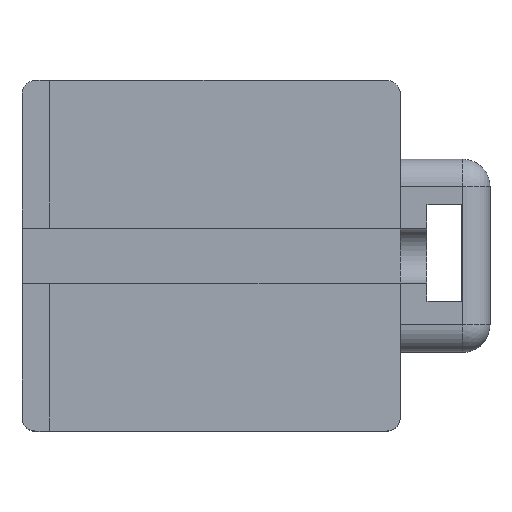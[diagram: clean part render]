
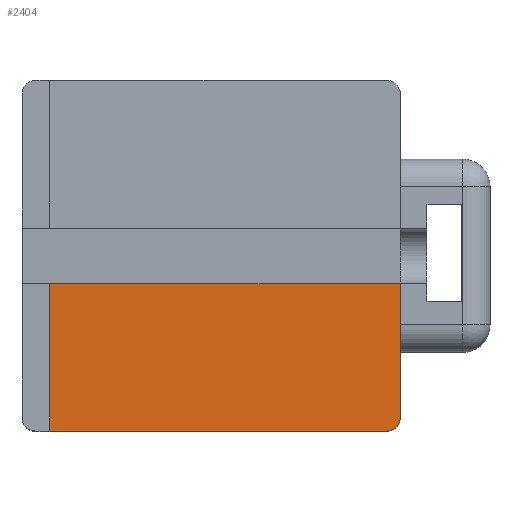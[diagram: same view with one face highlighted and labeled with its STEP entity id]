
A CAD part, top view. The second image highlights one B-rep face of the part: STEP entity #2404.
In plain terms, the highlighted planar face has unit normal (0, 0, 1).
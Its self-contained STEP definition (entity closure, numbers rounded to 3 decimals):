
#599 = PLANE('',#600);
#600 = AXIS2_PLACEMENT_3D('',#601,#602,#603);
#601 = CARTESIAN_POINT('',(4.864,-30.767,17.467));
#602 = DIRECTION('',(1.,0.,0.));
#603 = DIRECTION('',(0.,0.,1.));
#1413 = VERTEX_POINT('',#1414);
#1414 = CARTESIAN_POINT('',(4.864,-14.7,16.036));
#1428 = PLANE('',#1429);
#1429 = AXIS2_PLACEMENT_3D('',#1430,#1431,#1432);
#1430 = CARTESIAN_POINT('',(4.864,-14.7,14.));
#1431 = DIRECTION('',(0.,1.,0.));
#1432 = DIRECTION('',(0.,0.,1.));
#1440 = EDGE_CURVE('',#1441,#1413,#1443,.T.);
#1441 = VERTEX_POINT('',#1442);
#1442 = CARTESIAN_POINT('',(4.864,-24.4,16.036));
#1443 = SURFACE_CURVE('',#1444,(#1448,#1454),.PCURVE_S1.);
#1444 = LINE('',#1445,#1446);
#1445 = CARTESIAN_POINT('',(4.864,-28.084,16.036));
#1446 = VECTOR('',#1447,1.);
#1447 = DIRECTION('',(0.,1.,0.));
#1448 = PCURVE('',#599,#1449);
#1449 = DEFINITIONAL_REPRESENTATION('',(#1450),#1453);
#1450 = B_SPLINE_CURVE_WITH_KNOTS('',1,(#1451,#1452),.UNSPECIFIED.,.F.,
  .F.,(2,2),(0.144,30.624),.PIECEWISE_BEZIER_KNOTS.);
#1451 = CARTESIAN_POINT('',(-1.431,-2.827));
#1452 = CARTESIAN_POINT('',(-1.431,-33.307));
#1453 = ( GEOMETRIC_REPRESENTATION_CONTEXT(2) 
PARAMETRIC_REPRESENTATION_CONTEXT() REPRESENTATION_CONTEXT('2D SPACE',''
  ) );
#1454 = PCURVE('',#1455,#1460);
#1455 = PLANE('',#1456);
#1456 = AXIS2_PLACEMENT_3D('',#1457,#1458,#1459);
#1457 = CARTESIAN_POINT('',(-7.836,-25.4,16.036));
#1458 = DIRECTION('',(0.,0.,1.));
#1459 = DIRECTION('',(0.,-1.,0.));
#1460 = DEFINITIONAL_REPRESENTATION('',(#1461),#1464);
#1461 = B_SPLINE_CURVE_WITH_KNOTS('',1,(#1462,#1463),.UNSPECIFIED.,.F.,
  .F.,(2,2),(0.144,30.624),.PIECEWISE_BEZIER_KNOTS.);
#1462 = CARTESIAN_POINT('',(2.54,12.7));
#1463 = CARTESIAN_POINT('',(-27.94,12.7));
#1464 = ( GEOMETRIC_REPRESENTATION_CONTEXT(2) 
PARAMETRIC_REPRESENTATION_CONTEXT() REPRESENTATION_CONTEXT('2D SPACE',''
  ) );
#1482 = CYLINDRICAL_SURFACE('',#1483,1.);
#1483 = AXIS2_PLACEMENT_3D('',#1484,#1485,#1486);
#1484 = CARTESIAN_POINT('',(3.864,-24.4,9.686));
#1485 = DIRECTION('',(0.,0.,1.));
#1486 = DIRECTION('',(0.,-1.,0.));
#2361 = VERTEX_POINT('',#2362);
#2362 = CARTESIAN_POINT('',(-20.536,-14.7,16.036));
#2375 = PLANE('',#2376);
#2376 = AXIS2_PLACEMENT_3D('',#2377,#2378,#2379);
#2377 = CARTESIAN_POINT('',(-25.428,3.109,16.036));
#2378 = DIRECTION('',(0.,0.,1.));
#2379 = DIRECTION('',(1.,0.,0.));
#2386 = EDGE_CURVE('',#1413,#2361,#2387,.T.);
#2387 = SURFACE_CURVE('',#2388,(#2392,#2398),.PCURVE_S1.);
#2388 = LINE('',#2389,#2390);
#2389 = CARTESIAN_POINT('',(-1.486,-14.7,16.036));
#2390 = VECTOR('',#2391,1.);
#2391 = DIRECTION('',(-1.,0.,0.));
#2392 = PCURVE('',#1428,#2393);
#2393 = DEFINITIONAL_REPRESENTATION('',(#2394),#2397);
#2394 = B_SPLINE_CURVE_WITH_KNOTS('',1,(#2395,#2396),.UNSPECIFIED.,.F.,
  .F.,(2,2),(-8.89,21.59),.PIECEWISE_BEZIER_KNOTS.);
#2395 = CARTESIAN_POINT('',(2.036,2.54));
#2396 = CARTESIAN_POINT('',(2.036,-27.94));
#2397 = ( GEOMETRIC_REPRESENTATION_CONTEXT(2) 
PARAMETRIC_REPRESENTATION_CONTEXT() REPRESENTATION_CONTEXT('2D SPACE',''
  ) );
#2398 = PCURVE('',#1455,#2399);
#2399 = DEFINITIONAL_REPRESENTATION('',(#2400),#2403);
#2400 = B_SPLINE_CURVE_WITH_KNOTS('',1,(#2401,#2402),.UNSPECIFIED.,.F.,
  .F.,(2,2),(-8.89,21.59),.PIECEWISE_BEZIER_KNOTS.);
#2401 = CARTESIAN_POINT('',(-10.7,15.24));
#2402 = CARTESIAN_POINT('',(-10.7,-15.24));
#2403 = ( GEOMETRIC_REPRESENTATION_CONTEXT(2) 
PARAMETRIC_REPRESENTATION_CONTEXT() REPRESENTATION_CONTEXT('2D SPACE',''
  ) );
#2404 = ADVANCED_FACE('',(#2405),#1455,.T.);
#2405 = FACE_BOUND('',#2406,.T.);
#2406 = EDGE_LOOP('',(#2407,#2408,#2409,#2431,#2459));
#2407 = ORIENTED_EDGE('',*,*,#1440,.T.);
#2408 = ORIENTED_EDGE('',*,*,#2386,.T.);
#2409 = ORIENTED_EDGE('',*,*,#2410,.T.);
#2410 = EDGE_CURVE('',#2361,#2411,#2413,.T.);
#2411 = VERTEX_POINT('',#2412);
#2412 = CARTESIAN_POINT('',(-20.536,-25.4,16.036));
#2413 = SURFACE_CURVE('',#2414,(#2418,#2424),.PCURVE_S1.);
#2414 = LINE('',#2415,#2416);
#2415 = CARTESIAN_POINT('',(-20.536,-10.967,16.036));
#2416 = VECTOR('',#2417,1.);
#2417 = DIRECTION('',(0.,-1.,0.));
#2418 = PCURVE('',#1455,#2419);
#2419 = DEFINITIONAL_REPRESENTATION('',(#2420),#2423);
#2420 = B_SPLINE_CURVE_WITH_KNOTS('',1,(#2421,#2422),.UNSPECIFIED.,.F.,
  .F.,(2,2),(-13.507,16.973),.PIECEWISE_BEZIER_KNOTS.);
#2421 = CARTESIAN_POINT('',(-27.94,-12.7));
#2422 = CARTESIAN_POINT('',(2.54,-12.7));
#2423 = ( GEOMETRIC_REPRESENTATION_CONTEXT(2) 
PARAMETRIC_REPRESENTATION_CONTEXT() REPRESENTATION_CONTEXT('2D SPACE',''
  ) );
#2424 = PCURVE('',#2375,#2425);
#2425 = DEFINITIONAL_REPRESENTATION('',(#2426),#2430);
#2426 = LINE('',#2427,#2428);
#2427 = CARTESIAN_POINT('',(4.892,-14.076));
#2428 = VECTOR('',#2429,1.);
#2429 = DIRECTION('',(0.,-1.));
#2430 = ( GEOMETRIC_REPRESENTATION_CONTEXT(2) 
PARAMETRIC_REPRESENTATION_CONTEXT() REPRESENTATION_CONTEXT('2D SPACE',''
  ) );
#2431 = ORIENTED_EDGE('',*,*,#2432,.T.);
#2432 = EDGE_CURVE('',#2411,#2433,#2435,.T.);
#2433 = VERTEX_POINT('',#2434);
#2434 = CARTESIAN_POINT('',(3.864,-25.4,16.036));
#2435 = SURFACE_CURVE('',#2436,(#2440,#2447),.PCURVE_S1.);
#2436 = LINE('',#2437,#2438);
#2437 = CARTESIAN_POINT('',(-7.836,-25.4,16.036));
#2438 = VECTOR('',#2439,1.);
#2439 = DIRECTION('',(1.,0.,0.));
#2440 = PCURVE('',#1455,#2441);
#2441 = DEFINITIONAL_REPRESENTATION('',(#2442),#2446);
#2442 = LINE('',#2443,#2444);
#2443 = CARTESIAN_POINT('',(0.,0.));
#2444 = VECTOR('',#2445,1.);
#2445 = DIRECTION('',(0.,1.));
#2446 = ( GEOMETRIC_REPRESENTATION_CONTEXT(2) 
PARAMETRIC_REPRESENTATION_CONTEXT() REPRESENTATION_CONTEXT('2D SPACE',''
  ) );
#2447 = PCURVE('',#2448,#2453);
#2448 = PLANE('',#2449);
#2449 = AXIS2_PLACEMENT_3D('',#2450,#2451,#2452);
#2450 = CARTESIAN_POINT('',(-7.836,-25.4,-21.102));
#2451 = DIRECTION('',(0.,-1.,0.));
#2452 = DIRECTION('',(1.,0.,0.));
#2453 = DEFINITIONAL_REPRESENTATION('',(#2454),#2458);
#2454 = LINE('',#2455,#2456);
#2455 = CARTESIAN_POINT('',(0.,37.138));
#2456 = VECTOR('',#2457,1.);
#2457 = DIRECTION('',(1.,0.));
#2458 = ( GEOMETRIC_REPRESENTATION_CONTEXT(2) 
PARAMETRIC_REPRESENTATION_CONTEXT() REPRESENTATION_CONTEXT('2D SPACE',''
  ) );
#2459 = ORIENTED_EDGE('',*,*,#2460,.T.);
#2460 = EDGE_CURVE('',#2433,#1441,#2461,.T.);
#2461 = SURFACE_CURVE('',#2462,(#2467,#2474),.PCURVE_S1.);
#2462 = CIRCLE('',#2463,1.);
#2463 = AXIS2_PLACEMENT_3D('',#2464,#2465,#2466);
#2464 = CARTESIAN_POINT('',(3.864,-24.4,16.036));
#2465 = DIRECTION('',(0.,0.,1.));
#2466 = DIRECTION('',(0.,-1.,0.));
#2467 = PCURVE('',#1455,#2468);
#2468 = DEFINITIONAL_REPRESENTATION('',(#2469),#2473);
#2469 = CIRCLE('',#2470,1.);
#2470 = AXIS2_PLACEMENT_2D('',#2471,#2472);
#2471 = CARTESIAN_POINT('',(-1.,11.7));
#2472 = DIRECTION('',(1.,0.));
#2473 = ( GEOMETRIC_REPRESENTATION_CONTEXT(2) 
PARAMETRIC_REPRESENTATION_CONTEXT() REPRESENTATION_CONTEXT('2D SPACE',''
  ) );
#2474 = PCURVE('',#1482,#2475);
#2475 = DEFINITIONAL_REPRESENTATION('',(#2476),#2480);
#2476 = LINE('',#2477,#2478);
#2477 = CARTESIAN_POINT('',(0.,6.35));
#2478 = VECTOR('',#2479,1.);
#2479 = DIRECTION('',(1.,0.));
#2480 = ( GEOMETRIC_REPRESENTATION_CONTEXT(2) 
PARAMETRIC_REPRESENTATION_CONTEXT() REPRESENTATION_CONTEXT('2D SPACE',''
  ) );
